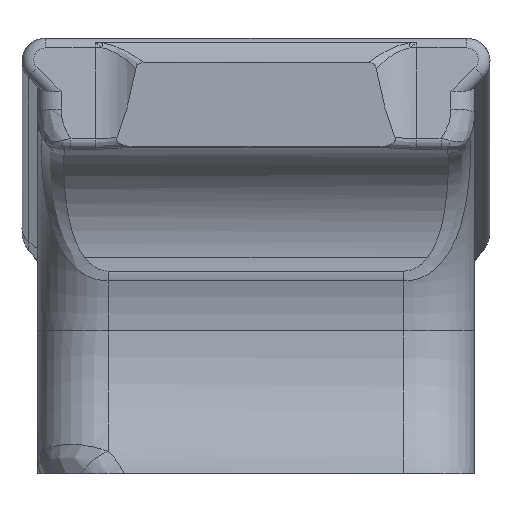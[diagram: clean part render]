
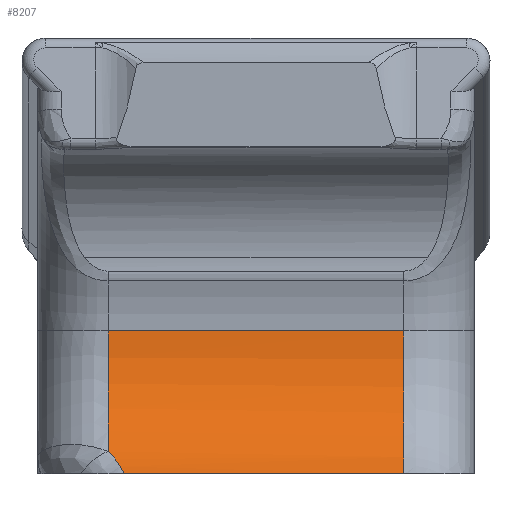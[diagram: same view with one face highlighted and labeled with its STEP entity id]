
A CAD part, left-side view. The second image highlights one B-rep face of the part: STEP entity #8207.
In plain terms, the highlighted cylindrical face has radius 14.287 mm (diameter 28.575 mm), a partial arc.
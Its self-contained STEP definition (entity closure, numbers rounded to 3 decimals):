
#255 = FACE_OUTER_BOUND ( 'NONE', #2342, .T. ) ;
#649 = VERTEX_POINT ( 'NONE', #2621 ) ;
#651 = VERTEX_POINT ( 'NONE', #6535 ) ;
#712 = ORIENTED_EDGE ( 'NONE', *, *, #2968, .T. ) ;
#818 = CARTESIAN_POINT ( 'NONE',  ( 84.171, -46.951, -13.516 ) ) ;
#819 = CARTESIAN_POINT ( 'NONE',  ( 84.671, -46.816, -13.206 ) ) ;
#832 = CARTESIAN_POINT ( 'NONE',  ( 85.113, -46.642, -12.89 ) ) ;
#838 = CARTESIAN_POINT ( 'NONE',  ( 85.515, -46.423, -12.573 ) ) ;
#848 = CARTESIAN_POINT ( 'NONE',  ( 85.529, -46.415, -12.562 ) ) ;
#849 = CARTESIAN_POINT ( 'NONE',  ( 85.556, -46.401, -12.541 ) ) ;
#870 = CARTESIAN_POINT ( 'NONE',  ( 85.595, -46.379, -12.51 ) ) ;
#879 = CARTESIAN_POINT ( 'NONE',  ( 85.685, -46.326, -12.437 ) ) ;
#881 = CARTESIAN_POINT ( 'NONE',  ( 85.761, -46.28, -12.375 ) ) ;
#886 = CARTESIAN_POINT ( 'NONE',  ( 85.909, -46.184, -12.251 ) ) ;
#889 = CARTESIAN_POINT ( 'NONE',  ( 86.005, -46.117, -12.169 ) ) ;
#909 = CARTESIAN_POINT ( 'NONE',  ( 86.281, -45.908, -11.925 ) ) ;
#943 = CARTESIAN_POINT ( 'NONE',  ( 86.612, -45.593, -11.611 ) ) ;
#951 = CARTESIAN_POINT ( 'NONE',  ( 86.453, -45.756, -11.766 ) ) ;
#1048 = VERTEX_POINT ( 'NONE', #2518 ) ;
#1163 = LINE ( 'NONE', #1972, #4605 ) ;
#1333 = CARTESIAN_POINT ( 'NONE',  ( 90.94, -45.593, -1.367 ) ) ;
#1465 = AXIS2_PLACEMENT_3D ( 'NONE', #3702, #4401, #2331 ) ;
#1955 = DIRECTION ( 'NONE',  ( 0., -1., 0. ) ) ;
#1972 = CARTESIAN_POINT ( 'NONE',  ( 84.171, -72.447, -13.516 ) ) ;
#2142 = VECTOR ( 'NONE', #5389, 1000. ) ;
#2331 = DIRECTION ( 'NONE',  ( 1., 0., 0. ) ) ;
#2342 = EDGE_LOOP ( 'NONE', ( #4100, #712, #7204, #3648, #2611 ) ) ;
#2518 = CARTESIAN_POINT ( 'NONE',  ( 84.171, -70.726, -13.516 ) ) ;
#2611 = ORIENTED_EDGE ( 'NONE', *, *, #3967, .T. ) ;
#2621 = CARTESIAN_POINT ( 'NONE',  ( 90.94, -70.726, -1.367 ) ) ;
#2653 = B_SPLINE_CURVE_WITH_KNOTS ( 'NONE', 3,
 ( #943, #951, #909, #889, #886, #881, #879, #870, #849, #848, #838, #832, #819, #818 ),
 .UNSPECIFIED., .F., .F.,
 ( 4, 2, 2, 1, 1, 2, 2, 4 ),
 ( 0., 0.25, 0.375, 0.437, 0.469, 0.484, 0.5, 1. ),
 .UNSPECIFIED. ) ;
#2968 = EDGE_CURVE ( 'NONE', #649, #5429, #6138, .T. ) ;
#3085 = DIRECTION ( 'NONE',  ( 1., 0., 0. ) ) ;
#3095 = DIRECTION ( 'NONE',  ( 0., 1., 0. ) ) ;
#3099 = VERTEX_POINT ( 'NONE', #5049 ) ;
#3109 = CARTESIAN_POINT ( 'NONE',  ( 76.653, -45.593, -1.367 ) ) ;
#3427 = EDGE_CURVE ( 'NONE', #1048, #649, #4505, .T. ) ;
#3510 = DIRECTION ( 'NONE',  ( 1., 0., 0. ) ) ;
#3522 = DIRECTION ( 'NONE',  ( 0., -1., 0. ) ) ;
#3523 = CARTESIAN_POINT ( 'NONE',  ( 76.653, -70.726, -1.367 ) ) ;
#3543 = EDGE_CURVE ( 'NONE', #5429, #3099, #7862, .T. ) ;
#3554 = AXIS2_PLACEMENT_3D ( 'NONE', #3109, #3095, #3085 ) ;
#3648 = ORIENTED_EDGE ( 'NONE', *, *, #4252, .T. ) ;
#3702 = CARTESIAN_POINT ( 'NONE',  ( 76.653, -72.447, -1.367 ) ) ;
#3967 = EDGE_CURVE ( 'NONE', #651, #1048, #1163, .T. ) ;
#3990 = AXIS2_PLACEMENT_3D ( 'NONE', #3523, #3522, #3510 ) ;
#4100 = ORIENTED_EDGE ( 'NONE', *, *, #3427, .T. ) ;
#4252 = EDGE_CURVE ( 'NONE', #3099, #651, #2653, .T. ) ;
#4401 = DIRECTION ( 'NONE',  ( 0., 1., 0. ) ) ;
#4505 = CIRCLE ( 'NONE', #3990, 14.288 ) ;
#4605 = VECTOR ( 'NONE', #1955, 1000. ) ;
#5049 = CARTESIAN_POINT ( 'NONE',  ( 86.612, -45.593, -11.611 ) ) ;
#5389 = DIRECTION ( 'NONE',  ( 0., 1., 0. ) ) ;
#5429 = VERTEX_POINT ( 'NONE', #1333 ) ;
#5739 = CARTESIAN_POINT ( 'NONE',  ( 90.94, -72.447, -1.367 ) ) ;
#6138 = LINE ( 'NONE', #5739, #2142 ) ;
#6535 = CARTESIAN_POINT ( 'NONE',  ( 84.171, -46.951, -13.516 ) ) ;
#6986 = CYLINDRICAL_SURFACE ( 'NONE', #1465, 14.288 ) ;
#7204 = ORIENTED_EDGE ( 'NONE', *, *, #3543, .T. ) ;
#7862 = CIRCLE ( 'NONE', #3554, 14.288 ) ;
#8207 = ADVANCED_FACE ( 'NONE', ( #255 ), #6986, .F. ) ;
